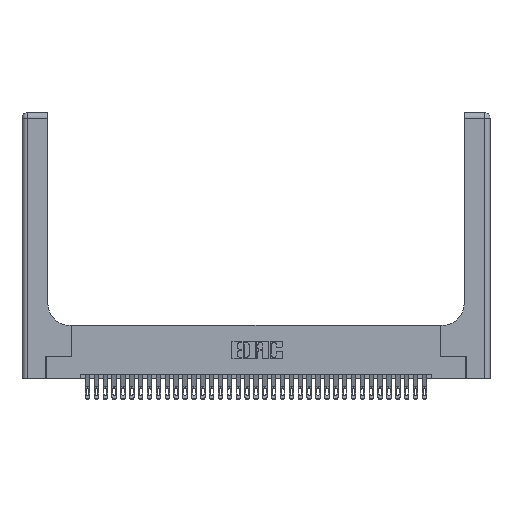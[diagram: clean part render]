
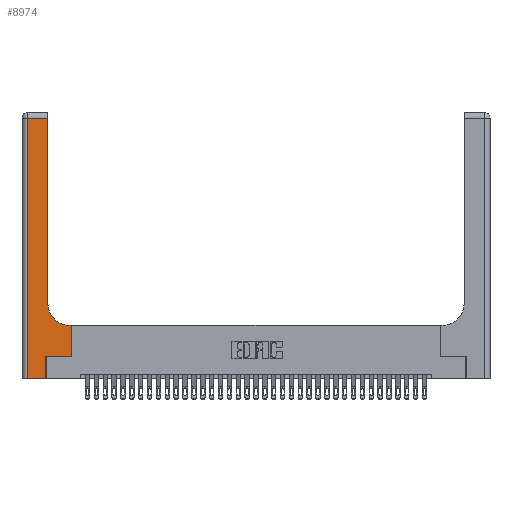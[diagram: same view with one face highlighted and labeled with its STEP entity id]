
A CAD part, top view. The second image highlights one B-rep face of the part: STEP entity #8974.
In plain terms, the highlighted planar face has unit normal (0, 0, 1).
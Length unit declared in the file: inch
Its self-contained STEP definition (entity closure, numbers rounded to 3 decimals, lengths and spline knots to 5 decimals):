
#969 = ORIENTED_EDGE ( 'NONE', *, *, #36368, .T. ) ;
#1169 = DIRECTION ( 'NONE',  ( 0., 0., -1. ) ) ;
#1358 = EDGE_CURVE ( 'NONE', #19349, #36187, #14689, .T. ) ;
#1513 = CARTESIAN_POINT ( 'NONE',  ( 0.2915, 0.85, 0.37 ) ) ;
#1564 = LINE ( 'NONE', #36346, #23644 ) ;
#2383 = ORIENTED_EDGE ( 'NONE', *, *, #35074, .T. ) ;
#2542 = VECTOR ( 'NONE', #19713, 39.37008 ) ;
#4539 = DIRECTION ( 'NONE',  ( 0., 1., 0. ) ) ;
#4578 = LINE ( 'NONE', #18622, #27092 ) ;
#4942 = ORIENTED_EDGE ( 'NONE', *, *, #1358, .T. ) ;
#5627 = AXIS2_PLACEMENT_3D ( 'NONE', #23813, #1169, #32241 ) ;
#5661 = EDGE_CURVE ( 'NONE', #36187, #27582, #23720, .T. ) ;
#5846 = FACE_OUTER_BOUND ( 'NONE', #36425, .T. ) ;
#6587 = LINE ( 'NONE', #14088, #13676 ) ;
#7757 = EDGE_CURVE ( 'NONE', #8222, #9306, #32741, .T. ) ;
#7893 = EDGE_CURVE ( 'NONE', #36114, #33727, #1564, .T. ) ;
#8165 = CARTESIAN_POINT ( 'NONE',  ( 0.5585, 0.6, 0.37 ) ) ;
#8222 = VERTEX_POINT ( 'NONE', #1513 ) ;
#8240 = ORIENTED_EDGE ( 'NONE', *, *, #22216, .T. ) ;
#8357 = DIRECTION ( 'NONE',  ( 1., 0., 0. ) ) ;
#8495 = ORIENTED_EDGE ( 'NONE', *, *, #34120, .T. ) ;
#8974 = ADVANCED_FACE ( 'NONE', ( #5846 ), #20488, .F. ) ;
#9076 = CARTESIAN_POINT ( 'NONE',  ( 0., 2.94, 0.37 ) ) ;
#9306 = VERTEX_POINT ( 'NONE', #21035 ) ;
#10688 = CARTESIAN_POINT ( 'NONE',  ( 0.5415, 0.6, 0.37 ) ) ;
#11032 = DIRECTION ( 'NONE',  ( 0., 1., 0. ) ) ;
#11696 = CARTESIAN_POINT ( 'NONE',  ( 0.269, 0., 0.37 ) ) ;
#13676 = VECTOR ( 'NONE', #11032, 39.37008 ) ;
#13822 = VECTOR ( 'NONE', #30407, 39.37008 ) ;
#14088 = CARTESIAN_POINT ( 'NONE',  ( 0.5585, 0.25, 0.37 ) ) ;
#14247 = VERTEX_POINT ( 'NONE', #10688 ) ;
#14478 = CARTESIAN_POINT ( 'NONE',  ( 0., 0., 0.37 ) ) ;
#14689 = LINE ( 'NONE', #27483, #13822 ) ;
#15742 = ORIENTED_EDGE ( 'NONE', *, *, #7893, .T. ) ;
#16856 = CARTESIAN_POINT ( 'NONE',  ( 0.2915, 0.6, 0.37 ) ) ;
#18099 = VERTEX_POINT ( 'NONE', #8165 ) ;
#18622 = CARTESIAN_POINT ( 'NONE',  ( 0.269, 0., 0.37 ) ) ;
#18815 = DIRECTION ( 'NONE',  ( 0., 1., 0. ) ) ;
#19349 = VERTEX_POINT ( 'NONE', #26359 ) ;
#19713 = DIRECTION ( 'NONE',  ( -1., 0., 0. ) ) ;
#20488 = PLANE ( 'NONE',  #32704 ) ;
#20847 = DIRECTION ( 'NONE',  ( -1., 0., 0. ) ) ;
#21035 = CARTESIAN_POINT ( 'NONE',  ( 0.2915, 2.94, 0.37 ) ) ;
#21605 = ORIENTED_EDGE ( 'NONE', *, *, #29921, .T. ) ;
#22216 = EDGE_CURVE ( 'NONE', #14247, #8222, #25469, .T. ) ;
#23206 = VECTOR ( 'NONE', #28906, 39.37008 ) ;
#23644 = VECTOR ( 'NONE', #30769, 39.37008 ) ;
#23720 = LINE ( 'NONE', #14478, #30272 ) ;
#23813 = CARTESIAN_POINT ( 'NONE',  ( 0.5415, 0.85, 0.37 ) ) ;
#25306 = VECTOR ( 'NONE', #18815, 39.37008 ) ;
#25469 = CIRCLE ( 'NONE', #5627, 0.25 ) ;
#25840 = LINE ( 'NONE', #9076, #23206 ) ;
#25940 = LINE ( 'NONE', #16856, #2542 ) ;
#26056 = CARTESIAN_POINT ( 'NONE',  ( 0., 3., 0.37 ) ) ;
#26359 = CARTESIAN_POINT ( 'NONE',  ( 0.06, 2.94, 0.37 ) ) ;
#26410 = DIRECTION ( 'NONE',  ( 0., 0., -1. ) ) ;
#27092 = VECTOR ( 'NONE', #4539, 39.37008 ) ;
#27483 = CARTESIAN_POINT ( 'NONE',  ( 0.06, 3., 0.37 ) ) ;
#27582 = VERTEX_POINT ( 'NONE', #11696 ) ;
#27761 = CARTESIAN_POINT ( 'NONE',  ( 0.5585, 0.25, 0.37 ) ) ;
#28105 = CARTESIAN_POINT ( 'NONE',  ( 0.269, 0.25, 0.37 ) ) ;
#28906 = DIRECTION ( 'NONE',  ( -1., 0., 0. ) ) ;
#29563 = ORIENTED_EDGE ( 'NONE', *, *, #5661, .T. ) ;
#29921 = EDGE_CURVE ( 'NONE', #33727, #18099, #6587, .T. ) ;
#30272 = VECTOR ( 'NONE', #8357, 39.37008 ) ;
#30407 = DIRECTION ( 'NONE',  ( 0., -1., 0. ) ) ;
#30769 = DIRECTION ( 'NONE',  ( 1., 0., 0. ) ) ;
#30792 = CARTESIAN_POINT ( 'NONE',  ( 0.06, 0., 0.37 ) ) ;
#32241 = DIRECTION ( 'NONE',  ( 1., 0., 0. ) ) ;
#32673 = CARTESIAN_POINT ( 'NONE',  ( 0.2915, 3., 0.37 ) ) ;
#32704 = AXIS2_PLACEMENT_3D ( 'NONE', #26056, #26410, #20847 ) ;
#32741 = LINE ( 'NONE', #32673, #25306 ) ;
#33727 = VERTEX_POINT ( 'NONE', #27761 ) ;
#33863 = ORIENTED_EDGE ( 'NONE', *, *, #7757, .T. ) ;
#34120 = EDGE_CURVE ( 'NONE', #27582, #36114, #4578, .T. ) ;
#35074 = EDGE_CURVE ( 'NONE', #18099, #14247, #25940, .T. ) ;
#36114 = VERTEX_POINT ( 'NONE', #28105 ) ;
#36187 = VERTEX_POINT ( 'NONE', #30792 ) ;
#36346 = CARTESIAN_POINT ( 'NONE',  ( 0.269, 0.25, 0.37 ) ) ;
#36368 = EDGE_CURVE ( 'NONE', #9306, #19349, #25840, .T. ) ;
#36425 = EDGE_LOOP ( 'NONE', ( #33863, #969, #4942, #29563, #8495, #15742, #21605, #2383, #8240 ) ) ;
